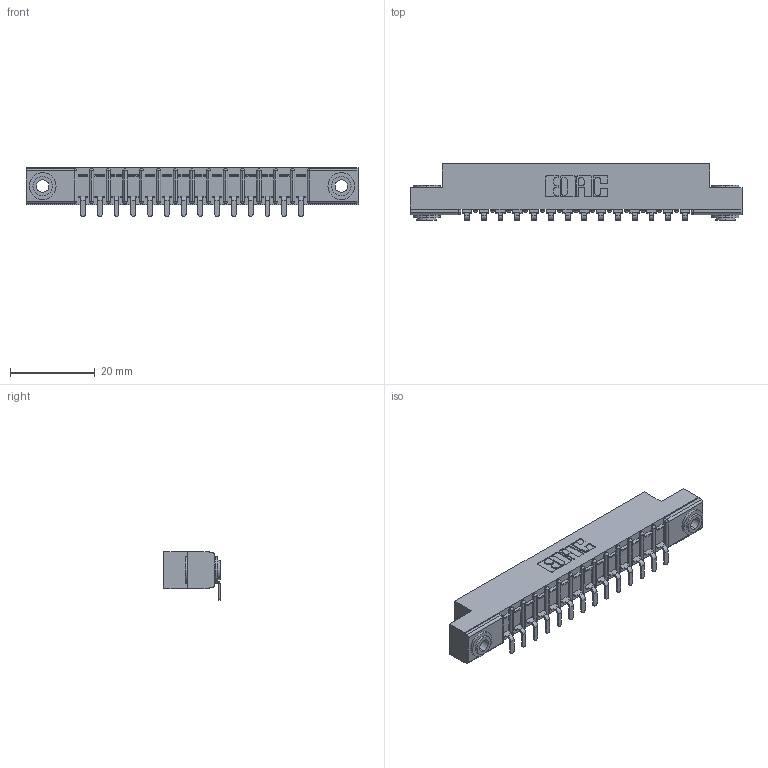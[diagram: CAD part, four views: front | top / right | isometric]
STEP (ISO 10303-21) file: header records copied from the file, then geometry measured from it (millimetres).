
FILE_DESCRIPTION (( 'STEP AP203' ), '1' );
FILE_NAME ('307-014-453-103.STEP', '2020-09-25T15:56:32', ( '' ), ( '' ), 'SwSTEP 2.0', 'SolidWorks 2020', '' );
FILE_SCHEMA (( 'CONFIG_CONTROL_DESIGN' ));
Length unit declared in the file: inch
Products named in the file (4): 307-290-002_553; 345-250-002_345-250-002-102; 307-014-453-103; 307 Part_.156 Dia Mounting Holes
Assembly tree (17 placements, depth 2):
  307-014-453-103
    307 Part_.156 Dia Mounting Holes
    307-290-002_553  x14
    345-250-002_345-250-002-102  x2
Bounding box: 78.49 x 13.36 x 11.51 mm (x, y, z)
Volume: 5178.5 mm3; surface area: 9222.3 mm2
Topology: 17 solids, 17 shells, 1277 faces, 3851 edges, 2522 vertices
Faces by surface type: plane 752, cylinder 487, sphere 30, cone 8
Entity records: 17373 total; most frequent: CARTESIAN_POINT 2905, ORIENTED_EDGE 2886, DIRECTION 2851, EDGE_CURVE 1443, LINE 1083, VECTOR 1083, VERTEX_POINT 938, AXIS2_PLACEMENT_3D 884
